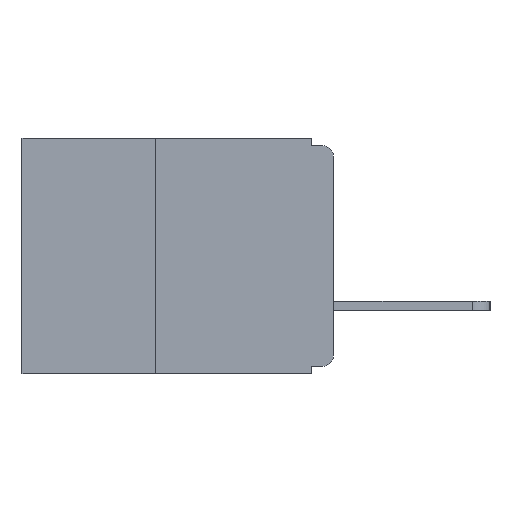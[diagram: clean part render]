
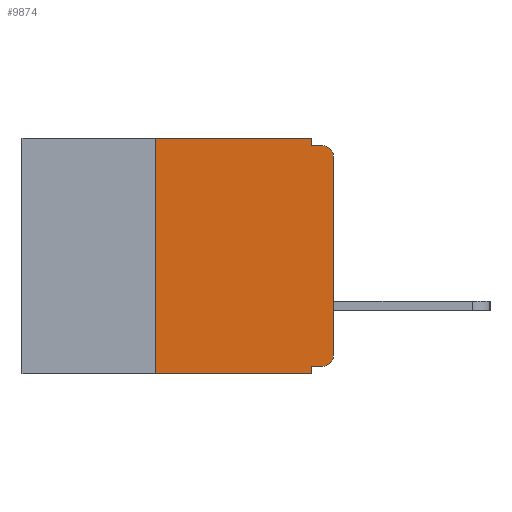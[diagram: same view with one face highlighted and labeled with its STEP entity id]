
A CAD part, left-side view. The second image highlights one B-rep face of the part: STEP entity #9874.
In plain terms, the highlighted planar face has unit normal (-1, 0, 0).
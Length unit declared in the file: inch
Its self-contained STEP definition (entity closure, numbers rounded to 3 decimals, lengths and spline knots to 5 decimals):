
#36 = CARTESIAN_POINT ( 'NONE',  ( 0., 0.031, -0.32 ) ) ;
#38 = EDGE_LOOP ( 'NONE', ( #5492, #6921, #552, #10231, #19580, #18280, #6814, #21161, #7950, #1330 ) ) ;
#174 = VERTEX_POINT ( 'NONE', #17899 ) ;
#235 = VECTOR ( 'NONE', #734, 39.37008 ) ;
#552 = ORIENTED_EDGE ( 'NONE', *, *, #16773, .F. ) ;
#734 = DIRECTION ( 'NONE',  ( 0., 1., 0. ) ) ;
#1330 = ORIENTED_EDGE ( 'NONE', *, *, #13439, .T. ) ;
#1467 = DIRECTION ( 'NONE',  ( 0., -1., 0. ) ) ;
#1519 = VECTOR ( 'NONE', #7227, 39.37008 ) ;
#2351 = CIRCLE ( 'NONE', #19208, 0.015 ) ;
#2629 = CARTESIAN_POINT ( 'NONE',  ( 0., 0., -0.305 ) ) ;
#2651 = VECTOR ( 'NONE', #5605, 39.37008 ) ;
#3193 = DIRECTION ( 'NONE',  ( 0., 0., 1. ) ) ;
#3584 = LINE ( 'NONE', #20183, #16797 ) ;
#3907 = DIRECTION ( 'NONE',  ( -1., 0., 0. ) ) ;
#4153 = LINE ( 'NONE', #5677, #235 ) ;
#4647 = VERTEX_POINT ( 'NONE', #6256 ) ;
#5441 = VERTEX_POINT ( 'NONE', #6800 ) ;
#5492 = ORIENTED_EDGE ( 'NONE', *, *, #10980, .T. ) ;
#5605 = DIRECTION ( 'NONE',  ( 0., 0., -1. ) ) ;
#5677 = CARTESIAN_POINT ( 'NONE',  ( 0., 0., -0.32 ) ) ;
#5688 = VECTOR ( 'NONE', #11549, 39.37008 ) ;
#5913 = PLANE ( 'NONE',  #8449 ) ;
#6018 = CARTESIAN_POINT ( 'NONE',  ( 0., 0.015, -0.01 ) ) ;
#6197 = LINE ( 'NONE', #21371, #5688 ) ;
#6256 = CARTESIAN_POINT ( 'NONE',  ( 0., 0.031, 0. ) ) ;
#6800 = CARTESIAN_POINT ( 'NONE',  ( 0., 0., -0.025 ) ) ;
#6814 = ORIENTED_EDGE ( 'NONE', *, *, #14232, .T. ) ;
#6921 = ORIENTED_EDGE ( 'NONE', *, *, #15423, .T. ) ;
#7018 = VECTOR ( 'NONE', #1467, 39.37008 ) ;
#7227 = DIRECTION ( 'NONE',  ( 0., -1., 0. ) ) ;
#7429 = VERTEX_POINT ( 'NONE', #36 ) ;
#7446 = CIRCLE ( 'NONE', #10717, 0.015 ) ;
#7790 = FACE_OUTER_BOUND ( 'NONE', #38, .T. ) ;
#7910 = CARTESIAN_POINT ( 'NONE',  ( 0., 0.015, -0.305 ) ) ;
#7950 = ORIENTED_EDGE ( 'NONE', *, *, #20322, .F. ) ;
#8078 = VERTEX_POINT ( 'NONE', #18621 ) ;
#8158 = EDGE_CURVE ( 'NONE', #4647, #174, #11489, .T. ) ;
#8449 = AXIS2_PLACEMENT_3D ( 'NONE', #17501, #20789, #10958 ) ;
#8642 = DIRECTION ( 'NONE',  ( 0., 0., 1. ) ) ;
#9454 = CARTESIAN_POINT ( 'NONE',  ( 0., 0.25, -0.33 ) ) ;
#9591 = DIRECTION ( 'NONE',  ( 0., 0., -1. ) ) ;
#9676 = CARTESIAN_POINT ( 'NONE',  ( 0., 0.25, 0. ) ) ;
#9874 = ADVANCED_FACE ( 'NONE', ( #7790 ), #5913, .F. ) ;
#10231 = ORIENTED_EDGE ( 'NONE', *, *, #8158, .F. ) ;
#10360 = LINE ( 'NONE', #18773, #1519 ) ;
#10717 = AXIS2_PLACEMENT_3D ( 'NONE', #13861, #3907, #15526 ) ;
#10727 = VERTEX_POINT ( 'NONE', #9676 ) ;
#10939 = LINE ( 'NONE', #21267, #7018 ) ;
#10958 = DIRECTION ( 'NONE',  ( 0., 0., -1. ) ) ;
#10980 = EDGE_CURVE ( 'NONE', #11560, #5441, #3584, .T. ) ;
#11140 = CARTESIAN_POINT ( 'NONE',  ( 0., 0., -0.01 ) ) ;
#11489 = LINE ( 'NONE', #15567, #2651 ) ;
#11549 = DIRECTION ( 'NONE',  ( 0., 0., -1. ) ) ;
#11560 = VERTEX_POINT ( 'NONE', #2629 ) ;
#11617 = VERTEX_POINT ( 'NONE', #9454 ) ;
#13136 = CARTESIAN_POINT ( 'NONE',  ( 0., 0.25, -0.33 ) ) ;
#13439 = EDGE_CURVE ( 'NONE', #20607, #11560, #2351, .T. ) ;
#13564 = EDGE_CURVE ( 'NONE', #11617, #10727, #17385, .T. ) ;
#13861 = CARTESIAN_POINT ( 'NONE',  ( 0., 0.015, -0.025 ) ) ;
#14056 = VECTOR ( 'NONE', #3193, 39.37008 ) ;
#14153 = VECTOR ( 'NONE', #17680, 39.37008 ) ;
#14232 = EDGE_CURVE ( 'NONE', #11617, #8078, #10360, .T. ) ;
#14659 = LINE ( 'NONE', #11140, #14153 ) ;
#14668 = CARTESIAN_POINT ( 'NONE',  ( 0., 0.015, -0.32 ) ) ;
#15423 = EDGE_CURVE ( 'NONE', #5441, #18956, #7446, .T. ) ;
#15526 = DIRECTION ( 'NONE',  ( 0., 0., -1. ) ) ;
#15567 = CARTESIAN_POINT ( 'NONE',  ( 0., 0.031, 0. ) ) ;
#16773 = EDGE_CURVE ( 'NONE', #174, #18956, #14659, .T. ) ;
#16797 = VECTOR ( 'NONE', #8642, 39.37008 ) ;
#17385 = LINE ( 'NONE', #13136, #14056 ) ;
#17501 = CARTESIAN_POINT ( 'NONE',  ( 0., 0.437, 0. ) ) ;
#17680 = DIRECTION ( 'NONE',  ( 0., -1., 0. ) ) ;
#17899 = CARTESIAN_POINT ( 'NONE',  ( 0., 0.031, -0.01 ) ) ;
#18280 = ORIENTED_EDGE ( 'NONE', *, *, #13564, .F. ) ;
#18621 = CARTESIAN_POINT ( 'NONE',  ( 0., 0.031, -0.33 ) ) ;
#18773 = CARTESIAN_POINT ( 'NONE',  ( 0., 0.437, -0.33 ) ) ;
#18956 = VERTEX_POINT ( 'NONE', #6018 ) ;
#19208 = AXIS2_PLACEMENT_3D ( 'NONE', #7910, #19466, #9591 ) ;
#19466 = DIRECTION ( 'NONE',  ( -1., 0., 0. ) ) ;
#19580 = ORIENTED_EDGE ( 'NONE', *, *, #19973, .F. ) ;
#19973 = EDGE_CURVE ( 'NONE', #10727, #4647, #10939, .T. ) ;
#20183 = CARTESIAN_POINT ( 'NONE',  ( 0., 0., 0. ) ) ;
#20322 = EDGE_CURVE ( 'NONE', #20607, #7429, #4153, .T. ) ;
#20607 = VERTEX_POINT ( 'NONE', #14668 ) ;
#20663 = EDGE_CURVE ( 'NONE', #7429, #8078, #6197, .T. ) ;
#20789 = DIRECTION ( 'NONE',  ( 1., 0., 0. ) ) ;
#21161 = ORIENTED_EDGE ( 'NONE', *, *, #20663, .F. ) ;
#21267 = CARTESIAN_POINT ( 'NONE',  ( 0., 0.437, 0. ) ) ;
#21371 = CARTESIAN_POINT ( 'NONE',  ( 0., 0.031, -0.33 ) ) ;
